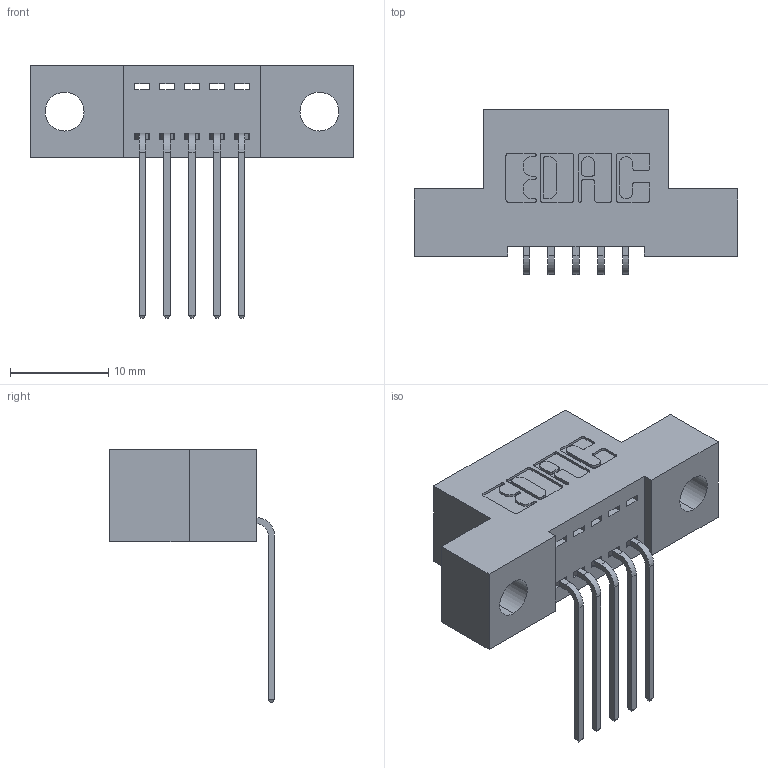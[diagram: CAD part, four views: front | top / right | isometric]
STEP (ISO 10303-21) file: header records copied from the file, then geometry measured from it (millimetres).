
FILE_DESCRIPTION (( 'STEP AP203' ), '1' );
FILE_NAME ('342-005-559-104.STEP', '2018-08-10T11:14:32', ( '' ), ( '' ), 'SwSTEP 2.0', 'SolidWorks 2016', '' );
FILE_SCHEMA (( 'CONFIG_CONTROL_DESIGN' ));
Length unit declared in the file: inch
Products named in the file (3): 342-005-559-104; 342 Part_.156 TH; 345-292-001_558 559 Tail - 1
Assembly tree (6 placements, depth 2):
  342-005-559-104
    342 Part_.156 TH
    345-292-001_558 559 Tail - 1  x5
Bounding box: 33.02 x 16.83 x 25.78 mm (x, y, z)
Volume: 2688.5 mm3; surface area: 3170.6 mm2
Topology: 6 solids, 6 shells, 410 faces, 1209 edges, 798 vertices
Faces by surface type: plane 286, cylinder 124
Entity records: 7797 total; most frequent: CARTESIAN_POINT 1357, ORIENTED_EDGE 1298, DIRECTION 1219, EDGE_CURVE 649, LINE 521, VECTOR 521, VERTEX_POINT 430, AXIS2_PLACEMENT_3D 349
